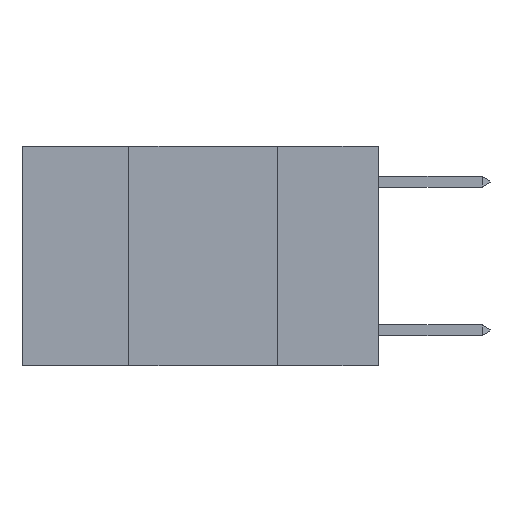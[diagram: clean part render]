
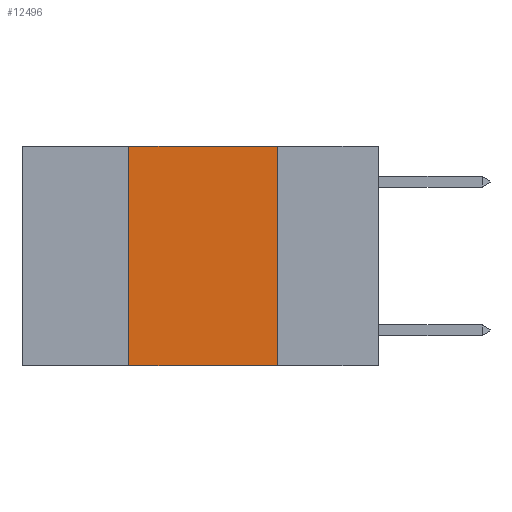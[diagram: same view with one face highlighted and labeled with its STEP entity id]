
A CAD part, left-side view. The second image highlights one B-rep face of the part: STEP entity #12496.
In plain terms, the highlighted planar face has unit normal (-1, 0, 0).
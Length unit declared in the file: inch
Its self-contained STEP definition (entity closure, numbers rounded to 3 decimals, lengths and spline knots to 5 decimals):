
#267 = ORIENTED_EDGE ( 'NONE', *, *, #1408, .F. ) ;
#865 = CARTESIAN_POINT ( 'NONE',  ( 0., 0.17, -0.37 ) ) ;
#1007 = LINE ( 'NONE', #11389, #10906 ) ;
#1403 = CARTESIAN_POINT ( 'NONE',  ( 0., 0.6, -0.37 ) ) ;
#1408 = EDGE_CURVE ( 'NONE', #5719, #3863, #1007, .T. ) ;
#1508 = EDGE_CURVE ( 'NONE', #2304, #5719, #6235, .T. ) ;
#2304 = VERTEX_POINT ( 'NONE', #6006 ) ;
#2393 = DIRECTION ( 'NONE',  ( 0., 0., -1. ) ) ;
#2475 = FACE_OUTER_BOUND ( 'NONE', #6612, .T. ) ;
#3376 = EDGE_CURVE ( 'NONE', #2304, #13671, #15670, .T. ) ;
#3780 = AXIS2_PLACEMENT_3D ( 'NONE', #3989, #3900, #2393 ) ;
#3863 = VERTEX_POINT ( 'NONE', #15973 ) ;
#3900 = DIRECTION ( 'NONE',  ( 1., 0., 0. ) ) ;
#3989 = CARTESIAN_POINT ( 'NONE',  ( 0., 0.6, 0. ) ) ;
#4071 = CARTESIAN_POINT ( 'NONE',  ( 0., 0.17, 0. ) ) ;
#4437 = VECTOR ( 'NONE', #9142, 39.37008 ) ;
#4490 = CARTESIAN_POINT ( 'NONE',  ( 0., 0.42, 0. ) ) ;
#5189 = ORIENTED_EDGE ( 'NONE', *, *, #8940, .F. ) ;
#5506 = VECTOR ( 'NONE', #10122, 39.37008 ) ;
#5719 = VERTEX_POINT ( 'NONE', #4490 ) ;
#6006 = CARTESIAN_POINT ( 'NONE',  ( 0., 0.42, -0.37 ) ) ;
#6235 = LINE ( 'NONE', #15016, #5506 ) ;
#6612 = EDGE_LOOP ( 'NONE', ( #5189, #267, #9558, #11555 ) ) ;
#7182 = DIRECTION ( 'NONE',  ( 0., -1., 0. ) ) ;
#8840 = DIRECTION ( 'NONE',  ( 0., -1., 0. ) ) ;
#8940 = EDGE_CURVE ( 'NONE', #3863, #13671, #14370, .T. ) ;
#9126 = PLANE ( 'NONE',  #3780 ) ;
#9142 = DIRECTION ( 'NONE',  ( 0., 0., -1. ) ) ;
#9558 = ORIENTED_EDGE ( 'NONE', *, *, #1508, .F. ) ;
#10122 = DIRECTION ( 'NONE',  ( 0., 0., 1. ) ) ;
#10906 = VECTOR ( 'NONE', #7182, 39.37008 ) ;
#11389 = CARTESIAN_POINT ( 'NONE',  ( 0., 0.6, 0. ) ) ;
#11555 = ORIENTED_EDGE ( 'NONE', *, *, #3376, .T. ) ;
#12496 = ADVANCED_FACE ( 'NONE', ( #2475 ), #9126, .F. ) ;
#13671 = VERTEX_POINT ( 'NONE', #865 ) ;
#13982 = VECTOR ( 'NONE', #8840, 39.37008 ) ;
#14370 = LINE ( 'NONE', #4071, #4437 ) ;
#15016 = CARTESIAN_POINT ( 'NONE',  ( 0., 0.42, 0. ) ) ;
#15670 = LINE ( 'NONE', #1403, #13982 ) ;
#15973 = CARTESIAN_POINT ( 'NONE',  ( 0., 0.17, 0. ) ) ;
